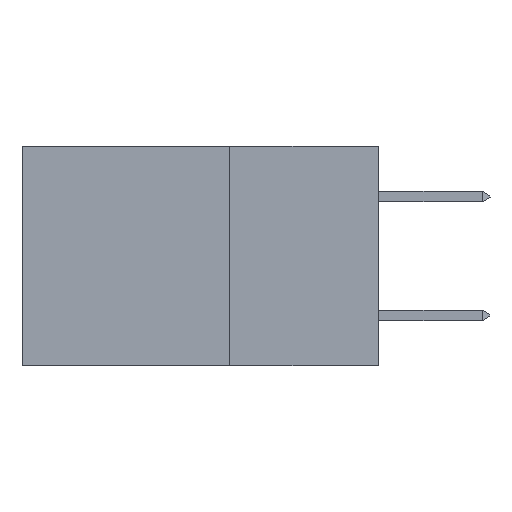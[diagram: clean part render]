
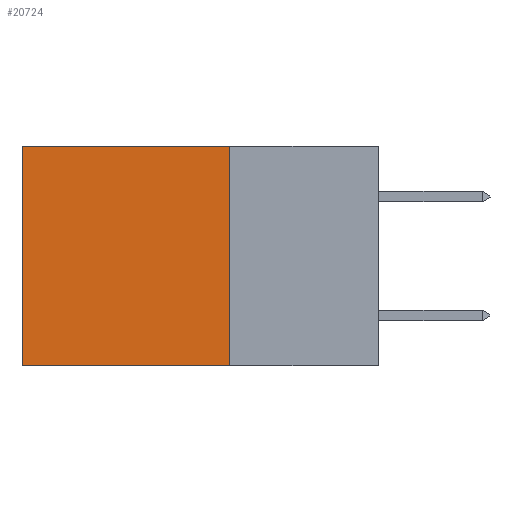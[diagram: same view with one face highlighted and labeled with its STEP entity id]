
A CAD part, left-side view. The second image highlights one B-rep face of the part: STEP entity #20724.
In plain terms, the highlighted planar face has unit normal (-1, 0, 0).
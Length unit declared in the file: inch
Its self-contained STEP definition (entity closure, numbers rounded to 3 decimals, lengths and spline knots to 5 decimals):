
#212 = ORIENTED_EDGE ( 'NONE', *, *, #15869, .F. ) ;
#269 = DIRECTION ( 'NONE',  ( 0., 1., 0. ) ) ;
#1489 = DIRECTION ( 'NONE',  ( 0., 0., -1. ) ) ;
#2009 = ORIENTED_EDGE ( 'NONE', *, *, #17522, .T. ) ;
#2046 = EDGE_CURVE ( 'NONE', #15761, #11660, #12155, .T. ) ;
#2424 = VECTOR ( 'NONE', #269, 39.37008 ) ;
#2487 = CARTESIAN_POINT ( 'NONE',  ( 0.298, 0.25, -0.37 ) ) ;
#3161 = PLANE ( 'NONE',  #21099 ) ;
#5425 = VECTOR ( 'NONE', #10688, 39.37008 ) ;
#5534 = ORIENTED_EDGE ( 'NONE', *, *, #5602, .F. ) ;
#5602 = EDGE_CURVE ( 'NONE', #5876, #11660, #19275, .T. ) ;
#5876 = VERTEX_POINT ( 'NONE', #2487 ) ;
#5921 = CARTESIAN_POINT ( 'NONE',  ( 0.298, 0.6, 0. ) ) ;
#7470 = CARTESIAN_POINT ( 'NONE',  ( 0.298, 0.25, 0. ) ) ;
#7608 = VECTOR ( 'NONE', #11203, 39.37008 ) ;
#8310 = DIRECTION ( 'NONE',  ( 0., 0., -1. ) ) ;
#8908 = VECTOR ( 'NONE', #8310, 39.37008 ) ;
#10688 = DIRECTION ( 'NONE',  ( 0., 1., 0. ) ) ;
#11203 = DIRECTION ( 'NONE',  ( 0., 0., -1. ) ) ;
#11252 = CARTESIAN_POINT ( 'NONE',  ( 0.298, 0.25, -0.37 ) ) ;
#11300 = ORIENTED_EDGE ( 'NONE', *, *, #2046, .T. ) ;
#11368 = CARTESIAN_POINT ( 'NONE',  ( 0.298, 0.6, -0.37 ) ) ;
#11660 = VERTEX_POINT ( 'NONE', #11368 ) ;
#11745 = DIRECTION ( 'NONE',  ( 1., 0., 0. ) ) ;
#12155 = LINE ( 'NONE', #5921, #7608 ) ;
#13303 = EDGE_LOOP ( 'NONE', ( #11300, #5534, #212, #2009 ) ) ;
#13465 = LINE ( 'NONE', #19929, #8908 ) ;
#15761 = VERTEX_POINT ( 'NONE', #19652 ) ;
#15869 = EDGE_CURVE ( 'NONE', #16206, #5876, #13465, .T. ) ;
#16206 = VERTEX_POINT ( 'NONE', #7470 ) ;
#16934 = FACE_OUTER_BOUND ( 'NONE', #13303, .T. ) ;
#17522 = EDGE_CURVE ( 'NONE', #16206, #15761, #20253, .T. ) ;
#18829 = CARTESIAN_POINT ( 'NONE',  ( 0.298, 0.25, 0. ) ) ;
#19275 = LINE ( 'NONE', #11252, #5425 ) ;
#19652 = CARTESIAN_POINT ( 'NONE',  ( 0.298, 0.6, 0. ) ) ;
#19929 = CARTESIAN_POINT ( 'NONE',  ( 0.298, 0.25, 0. ) ) ;
#19931 = CARTESIAN_POINT ( 'NONE',  ( 0.298, 0.25, 0. ) ) ;
#20253 = LINE ( 'NONE', #18829, #2424 ) ;
#20724 = ADVANCED_FACE ( 'NONE', ( #16934 ), #3161, .F. ) ;
#21099 = AXIS2_PLACEMENT_3D ( 'NONE', #19931, #11745, #1489 ) ;
